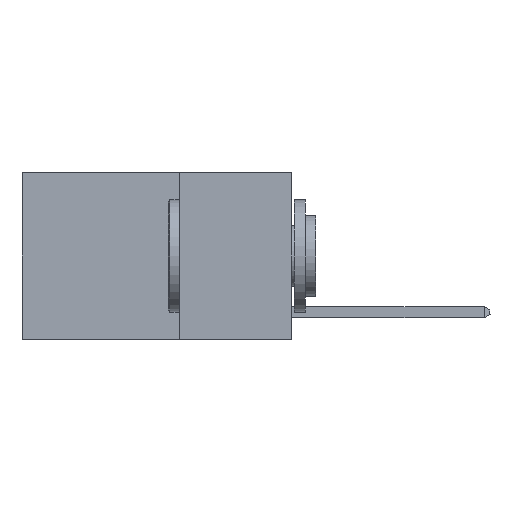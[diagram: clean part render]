
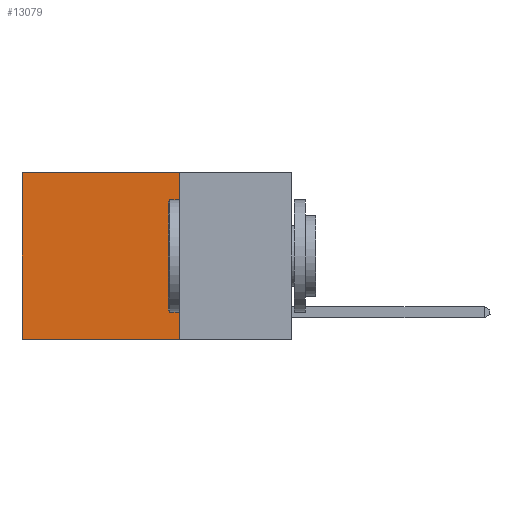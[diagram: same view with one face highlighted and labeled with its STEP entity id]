
A CAD part, left-side view. The second image highlights one B-rep face of the part: STEP entity #13079.
In plain terms, the highlighted planar face has unit normal (-1, 0, 0).
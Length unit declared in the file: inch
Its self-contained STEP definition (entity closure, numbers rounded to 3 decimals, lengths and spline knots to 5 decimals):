
#460 = AXIS2_PLACEMENT_3D ( 'NONE', #17561, #8798, #3611 ) ;
#785 = DIRECTION ( 'NONE',  ( 0., 1., 0. ) ) ;
#1713 = CARTESIAN_POINT ( 'NONE',  ( 0.2625, 0.25, 0. ) ) ;
#2368 = LINE ( 'NONE', #5891, #9738 ) ;
#3004 = FACE_OUTER_BOUND ( 'NONE', #17159, .T. ) ;
#3055 = EDGE_CURVE ( 'NONE', #7600, #13747, #11296, .T. ) ;
#3611 = DIRECTION ( 'NONE',  ( 0., 0., -1. ) ) ;
#3655 = ORIENTED_EDGE ( 'NONE', *, *, #5461, .F. ) ;
#3950 = ORIENTED_EDGE ( 'NONE', *, *, #6228, .F. ) ;
#4121 = CARTESIAN_POINT ( 'NONE',  ( 0.2625, 0.25, 0. ) ) ;
#4344 = PLANE ( 'NONE',  #460 ) ;
#4898 = CARTESIAN_POINT ( 'NONE',  ( 0.2625, 0.6, -0.37 ) ) ;
#5329 = VERTEX_POINT ( 'NONE', #4898 ) ;
#5461 = EDGE_CURVE ( 'NONE', #6572, #5329, #5916, .T. ) ;
#5891 = CARTESIAN_POINT ( 'NONE',  ( 0.2625, 0.6, 0. ) ) ;
#5916 = LINE ( 'NONE', #6622, #12839 ) ;
#6228 = EDGE_CURVE ( 'NONE', #7600, #6572, #14893, .T. ) ;
#6572 = VERTEX_POINT ( 'NONE', #12295 ) ;
#6609 = CARTESIAN_POINT ( 'NONE',  ( 0.2625, 0.6, 0. ) ) ;
#6622 = CARTESIAN_POINT ( 'NONE',  ( 0.2625, 0.25, -0.37 ) ) ;
#6845 = ORIENTED_EDGE ( 'NONE', *, *, #14094, .T. ) ;
#7053 = VECTOR ( 'NONE', #15869, 39.37008 ) ;
#7600 = VERTEX_POINT ( 'NONE', #1713 ) ;
#8798 = DIRECTION ( 'NONE',  ( 1., 0., 0. ) ) ;
#9738 = VECTOR ( 'NONE', #11803, 39.37008 ) ;
#9979 = DIRECTION ( 'NONE',  ( 0., 1., 0. ) ) ;
#11296 = LINE ( 'NONE', #15811, #18599 ) ;
#11803 = DIRECTION ( 'NONE',  ( 0., 0., -1. ) ) ;
#12295 = CARTESIAN_POINT ( 'NONE',  ( 0.2625, 0.25, -0.37 ) ) ;
#12839 = VECTOR ( 'NONE', #785, 39.37008 ) ;
#13079 = ADVANCED_FACE ( 'NONE', ( #3004 ), #4344, .F. ) ;
#13747 = VERTEX_POINT ( 'NONE', #6609 ) ;
#13784 = ORIENTED_EDGE ( 'NONE', *, *, #3055, .T. ) ;
#14094 = EDGE_CURVE ( 'NONE', #13747, #5329, #2368, .T. ) ;
#14893 = LINE ( 'NONE', #4121, #7053 ) ;
#15811 = CARTESIAN_POINT ( 'NONE',  ( 0.2625, 0.25, 0. ) ) ;
#15869 = DIRECTION ( 'NONE',  ( 0., 0., -1. ) ) ;
#17159 = EDGE_LOOP ( 'NONE', ( #6845, #3655, #3950, #13784 ) ) ;
#17561 = CARTESIAN_POINT ( 'NONE',  ( 0.2625, 0.25, 0. ) ) ;
#18599 = VECTOR ( 'NONE', #9979, 39.37008 ) ;
